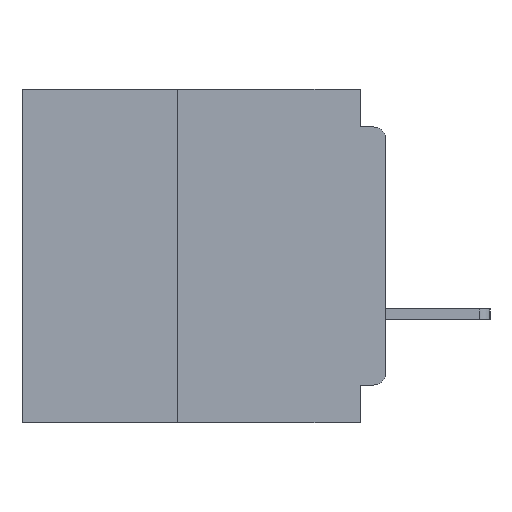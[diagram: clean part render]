
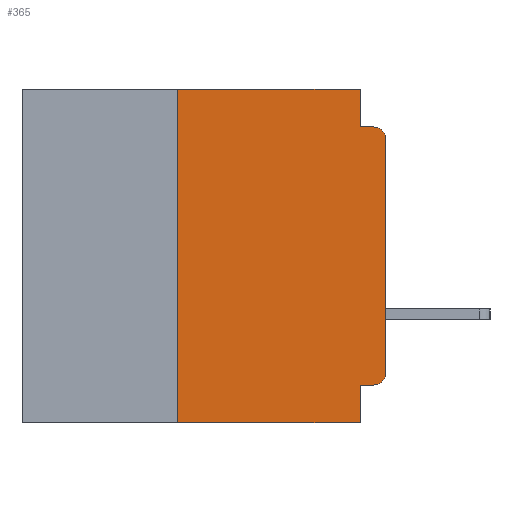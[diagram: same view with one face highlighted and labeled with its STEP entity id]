
A CAD part, left-side view. The second image highlights one B-rep face of the part: STEP entity #365.
In plain terms, the highlighted planar face has unit normal (-1, 0, 0).
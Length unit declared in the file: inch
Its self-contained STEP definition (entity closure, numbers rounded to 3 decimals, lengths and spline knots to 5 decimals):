
#365 = ADVANCED_FACE ( 'NONE', ( #24080 ), #27611, .F. ) ;
#415 = DIRECTION ( 'NONE',  ( -1., 0., 0. ) ) ;
#636 = ORIENTED_EDGE ( 'NONE', *, *, #14163, .T. ) ;
#1403 = EDGE_CURVE ( 'NONE', #15980, #9293, #33644, .T. ) ;
#1471 = AXIS2_PLACEMENT_3D ( 'NONE', #19004, #18252, #18378 ) ;
#2390 = VECTOR ( 'NONE', #26099, 39.37008 ) ;
#2994 = ORIENTED_EDGE ( 'NONE', *, *, #7994, .T. ) ;
#2998 = VECTOR ( 'NONE', #17093, 39.37008 ) ;
#3791 = VERTEX_POINT ( 'NONE', #5475 ) ;
#5269 = EDGE_LOOP ( 'NONE', ( #636, #2994, #27015, #12517, #19927, #32517, #16621, #34898, #24077, #22226 ) ) ;
#5475 = CARTESIAN_POINT ( 'NONE',  ( 0., 0.015, -0.045 ) ) ;
#5681 = CARTESIAN_POINT ( 'NONE',  ( 0., 0., -0.34 ) ) ;
#6711 = VERTEX_POINT ( 'NONE', #33763 ) ;
#6737 = CARTESIAN_POINT ( 'NONE',  ( 0., 0., -0.045 ) ) ;
#7327 = VERTEX_POINT ( 'NONE', #5681 ) ;
#7994 = EDGE_CURVE ( 'NONE', #16853, #3791, #9694, .T. ) ;
#8315 = VECTOR ( 'NONE', #30210, 39.37008 ) ;
#8978 = LINE ( 'NONE', #6737, #10766 ) ;
#9293 = VERTEX_POINT ( 'NONE', #17074 ) ;
#9694 = CIRCLE ( 'NONE', #13870, 0.015 ) ;
#9856 = AXIS2_PLACEMENT_3D ( 'NONE', #17781, #415, #20625 ) ;
#9955 = DIRECTION ( 'NONE',  ( 0., 0., -1. ) ) ;
#10062 = LINE ( 'NONE', #25194, #24258 ) ;
#10441 = CARTESIAN_POINT ( 'NONE',  ( 0., 0.031, -0.4 ) ) ;
#10766 = VECTOR ( 'NONE', #23810, 39.37008 ) ;
#11109 = DIRECTION ( 'NONE',  ( 0., -1., 0. ) ) ;
#11205 = VERTEX_POINT ( 'NONE', #31624 ) ;
#11618 = CARTESIAN_POINT ( 'NONE',  ( 0., 0.015, -0.06 ) ) ;
#11906 = EDGE_CURVE ( 'NONE', #11205, #30643, #16273, .T. ) ;
#12089 = LINE ( 'NONE', #34858, #25336 ) ;
#12517 = ORIENTED_EDGE ( 'NONE', *, *, #11906, .F. ) ;
#13870 = AXIS2_PLACEMENT_3D ( 'NONE', #11618, #31343, #14468 ) ;
#14163 = EDGE_CURVE ( 'NONE', #7327, #16853, #32439, .T. ) ;
#14468 = DIRECTION ( 'NONE',  ( 0., 0., -1. ) ) ;
#14654 = EDGE_CURVE ( 'NONE', #30643, #3791, #8978, .T. ) ;
#15469 = VERTEX_POINT ( 'NONE', #22105 ) ;
#15880 = DIRECTION ( 'NONE',  ( 0., 1., 0. ) ) ;
#15980 = VERTEX_POINT ( 'NONE', #30077 ) ;
#16273 = LINE ( 'NONE', #18371, #30425 ) ;
#16621 = ORIENTED_EDGE ( 'NONE', *, *, #35202, .T. ) ;
#16853 = VERTEX_POINT ( 'NONE', #34468 ) ;
#17074 = CARTESIAN_POINT ( 'NONE',  ( 0., 0.25, 0. ) ) ;
#17093 = DIRECTION ( 'NONE',  ( 0., 0., 1. ) ) ;
#17659 = VECTOR ( 'NONE', #15880, 39.37008 ) ;
#17769 = EDGE_CURVE ( 'NONE', #9293, #11205, #12089, .T. ) ;
#17781 = CARTESIAN_POINT ( 'NONE',  ( 0., 0.015, -0.34 ) ) ;
#18252 = DIRECTION ( 'NONE',  ( 1., 0., 0. ) ) ;
#18363 = EDGE_CURVE ( 'NONE', #19244, #7327, #20498, .T. ) ;
#18371 = CARTESIAN_POINT ( 'NONE',  ( 0., 0.031, 0. ) ) ;
#18378 = DIRECTION ( 'NONE',  ( 0., 0., -1. ) ) ;
#19004 = CARTESIAN_POINT ( 'NONE',  ( 0., 0.437, 0. ) ) ;
#19244 = VERTEX_POINT ( 'NONE', #35513 ) ;
#19927 = ORIENTED_EDGE ( 'NONE', *, *, #17769, .F. ) ;
#20498 = CIRCLE ( 'NONE', #9856, 0.015 ) ;
#20512 = EDGE_CURVE ( 'NONE', #19244, #6711, #26045, .T. ) ;
#20581 = EDGE_CURVE ( 'NONE', #6711, #15469, #30886, .T. ) ;
#20625 = DIRECTION ( 'NONE',  ( 0., 0., -1. ) ) ;
#20793 = DIRECTION ( 'NONE',  ( 0., -1., 0. ) ) ;
#22105 = CARTESIAN_POINT ( 'NONE',  ( 0., 0.031, -0.4 ) ) ;
#22226 = ORIENTED_EDGE ( 'NONE', *, *, #18363, .T. ) ;
#23810 = DIRECTION ( 'NONE',  ( 0., -1., 0. ) ) ;
#24077 = ORIENTED_EDGE ( 'NONE', *, *, #20512, .F. ) ;
#24080 = FACE_OUTER_BOUND ( 'NONE', #5269, .T. ) ;
#24258 = VECTOR ( 'NONE', #11109, 39.37008 ) ;
#25194 = CARTESIAN_POINT ( 'NONE',  ( 0., 0.437, -0.4 ) ) ;
#25336 = VECTOR ( 'NONE', #20793, 39.37008 ) ;
#25978 = CARTESIAN_POINT ( 'NONE',  ( 0., 0.25, -0.4 ) ) ;
#26045 = LINE ( 'NONE', #27117, #17659 ) ;
#26099 = DIRECTION ( 'NONE',  ( 0., 0., 1. ) ) ;
#26728 = CARTESIAN_POINT ( 'NONE',  ( 0., 0.031, -0.045 ) ) ;
#27015 = ORIENTED_EDGE ( 'NONE', *, *, #14654, .F. ) ;
#27117 = CARTESIAN_POINT ( 'NONE',  ( 0., 0., -0.355 ) ) ;
#27611 = PLANE ( 'NONE',  #1471 ) ;
#30077 = CARTESIAN_POINT ( 'NONE',  ( 0., 0.25, -0.4 ) ) ;
#30210 = DIRECTION ( 'NONE',  ( 0., 0., -1. ) ) ;
#30425 = VECTOR ( 'NONE', #9955, 39.37008 ) ;
#30643 = VERTEX_POINT ( 'NONE', #26728 ) ;
#30886 = LINE ( 'NONE', #10441, #8315 ) ;
#31343 = DIRECTION ( 'NONE',  ( -1., 0., 0. ) ) ;
#31624 = CARTESIAN_POINT ( 'NONE',  ( 0., 0.031, 0. ) ) ;
#32439 = LINE ( 'NONE', #33988, #2998 ) ;
#32517 = ORIENTED_EDGE ( 'NONE', *, *, #1403, .F. ) ;
#33644 = LINE ( 'NONE', #25978, #2390 ) ;
#33763 = CARTESIAN_POINT ( 'NONE',  ( 0., 0.031, -0.355 ) ) ;
#33988 = CARTESIAN_POINT ( 'NONE',  ( 0., 0., 0. ) ) ;
#34468 = CARTESIAN_POINT ( 'NONE',  ( 0., 0., -0.06 ) ) ;
#34858 = CARTESIAN_POINT ( 'NONE',  ( 0., 0.437, 0. ) ) ;
#34898 = ORIENTED_EDGE ( 'NONE', *, *, #20581, .F. ) ;
#35202 = EDGE_CURVE ( 'NONE', #15980, #15469, #10062, .T. ) ;
#35513 = CARTESIAN_POINT ( 'NONE',  ( 0., 0.015, -0.355 ) ) ;
